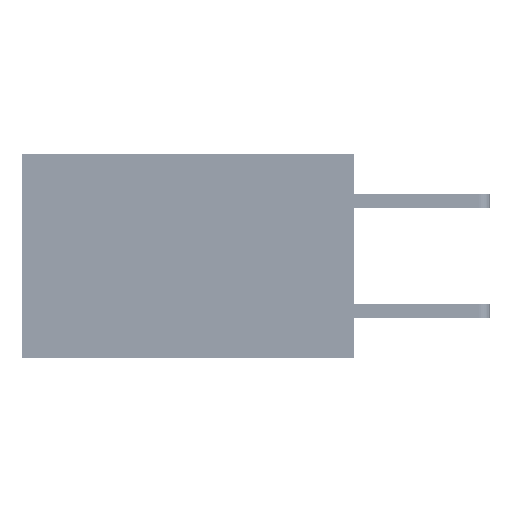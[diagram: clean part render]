
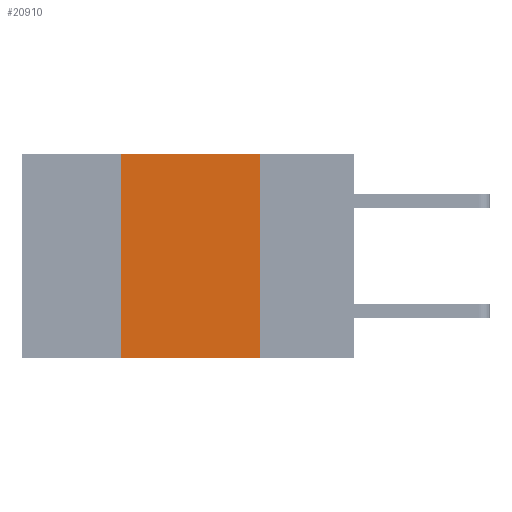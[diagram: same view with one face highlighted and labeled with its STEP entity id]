
A CAD part, left-side view. The second image highlights one B-rep face of the part: STEP entity #20910.
In plain terms, the highlighted planar face has unit normal (-1, 0, 0).
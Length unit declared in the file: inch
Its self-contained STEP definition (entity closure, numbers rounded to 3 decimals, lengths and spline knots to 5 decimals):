
#1754 = LINE ( 'NONE', #7678, #35265 ) ;
#2583 = DIRECTION ( 'NONE',  ( 1., 0., 0. ) ) ;
#3236 = DIRECTION ( 'NONE',  ( 0., 0., -1. ) ) ;
#7662 = AXIS2_PLACEMENT_3D ( 'NONE', #29920, #2583, #3236 ) ;
#7678 = CARTESIAN_POINT ( 'NONE',  ( 0., 0.17, 0. ) ) ;
#8533 = DIRECTION ( 'NONE',  ( 0., 0., 1. ) ) ;
#8822 = DIRECTION ( 'NONE',  ( 0., -1., 0. ) ) ;
#9096 = CARTESIAN_POINT ( 'NONE',  ( 0., 0.42, 0. ) ) ;
#9597 = PLANE ( 'NONE',  #7662 ) ;
#10487 = VECTOR ( 'NONE', #8822, 39.37008 ) ;
#10879 = LINE ( 'NONE', #35113, #29982 ) ;
#13085 = FACE_OUTER_BOUND ( 'NONE', #15525, .T. ) ;
#13094 = EDGE_CURVE ( 'NONE', #28436, #23494, #41122, .T. ) ;
#13370 = VECTOR ( 'NONE', #8533, 39.37008 ) ;
#15157 = LINE ( 'NONE', #18666, #10487 ) ;
#15525 = EDGE_LOOP ( 'NONE', ( #27985, #23638, #25631, #21116 ) ) ;
#18666 = CARTESIAN_POINT ( 'NONE',  ( 0., 0.6, 0. ) ) ;
#19110 = CARTESIAN_POINT ( 'NONE',  ( 0., 0.17, 0. ) ) ;
#19927 = VERTEX_POINT ( 'NONE', #19110 ) ;
#20910 = ADVANCED_FACE ( 'NONE', ( #13085 ), #9597, .F. ) ;
#21116 = ORIENTED_EDGE ( 'NONE', *, *, #38147, .T. ) ;
#23494 = VERTEX_POINT ( 'NONE', #9096 ) ;
#23638 = ORIENTED_EDGE ( 'NONE', *, *, #41153, .F. ) ;
#24722 = CARTESIAN_POINT ( 'NONE',  ( 0., 0.42, 0. ) ) ;
#24863 = CARTESIAN_POINT ( 'NONE',  ( 0., 0.17, -0.37 ) ) ;
#25631 = ORIENTED_EDGE ( 'NONE', *, *, #13094, .F. ) ;
#27184 = VERTEX_POINT ( 'NONE', #24863 ) ;
#27985 = ORIENTED_EDGE ( 'NONE', *, *, #35924, .F. ) ;
#28436 = VERTEX_POINT ( 'NONE', #39060 ) ;
#29920 = CARTESIAN_POINT ( 'NONE',  ( 0., 0.6, 0. ) ) ;
#29982 = VECTOR ( 'NONE', #41037, 39.37008 ) ;
#35113 = CARTESIAN_POINT ( 'NONE',  ( 0., 0.6, -0.37 ) ) ;
#35265 = VECTOR ( 'NONE', #41776, 39.37008 ) ;
#35924 = EDGE_CURVE ( 'NONE', #19927, #27184, #1754, .T. ) ;
#38147 = EDGE_CURVE ( 'NONE', #28436, #27184, #10879, .T. ) ;
#39060 = CARTESIAN_POINT ( 'NONE',  ( 0., 0.42, -0.37 ) ) ;
#41037 = DIRECTION ( 'NONE',  ( 0., -1., 0. ) ) ;
#41122 = LINE ( 'NONE', #24722, #13370 ) ;
#41153 = EDGE_CURVE ( 'NONE', #23494, #19927, #15157, .T. ) ;
#41776 = DIRECTION ( 'NONE',  ( 0., 0., -1. ) ) ;
